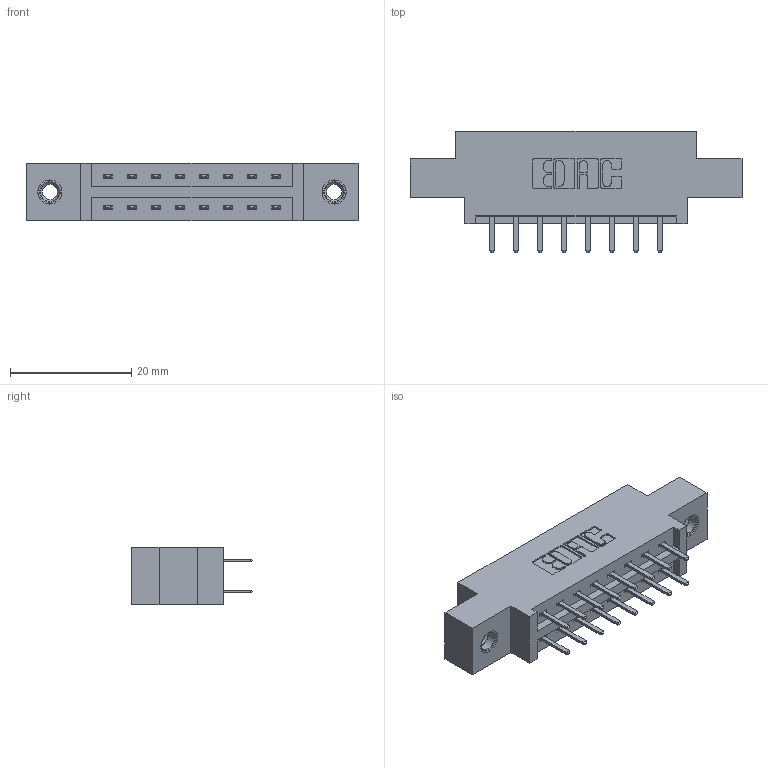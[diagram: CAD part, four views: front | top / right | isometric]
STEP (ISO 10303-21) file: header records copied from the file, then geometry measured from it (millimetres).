
FILE_DESCRIPTION (( 'STEP AP203' ), '1' );
FILE_NAME ('387-016-520-807.STEP', '2018-09-11T08:59:35', ( '' ), ( '' ), 'SwSTEP 2.0', 'SolidWorks 2016', '' );
FILE_SCHEMA (( 'CONFIG_CONTROL_DESIGN' ));
Length unit declared in the file: inch
Products named in the file (4): 387-016-520-807; 337 Part_0.170 Offset - 0.156 Dia-TI; 345-292-001_345-293-120; 345-250-001_345-250-005-103
Assembly tree (19 placements, depth 2):
  387-016-520-807
    337 Part_0.170 Offset - 0.156 Dia-TI
    345-292-001_345-293-120  x16
    345-250-001_345-250-005-103  x2
Bounding box: 54.71 x 20.02 x 9.4 mm (x, y, z)
Volume: 5175.3 mm3; surface area: 5644.2 mm2
Topology: 19 solids, 19 shells, 1106 faces, 3163 edges, 2058 vertices
Faces by surface type: plane 746, cylinder 344, cone 12, torus 4
Entity records: 12032 total; most frequent: CARTESIAN_POINT 2049, ORIENTED_EDGE 1966, DIRECTION 1825, EDGE_CURVE 983, LINE 831, VECTOR 831, VERTEX_POINT 648, AXIS2_PLACEMENT_3D 497
